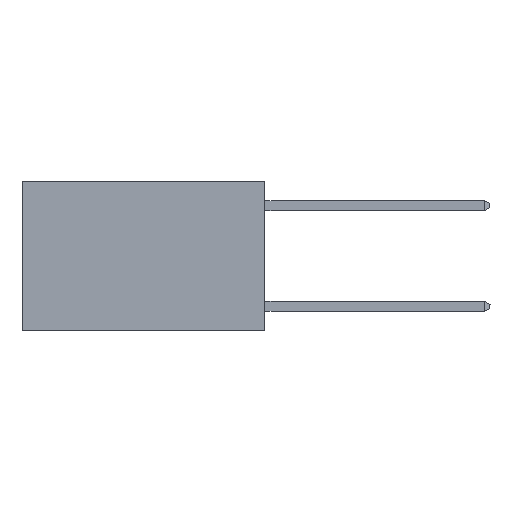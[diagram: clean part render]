
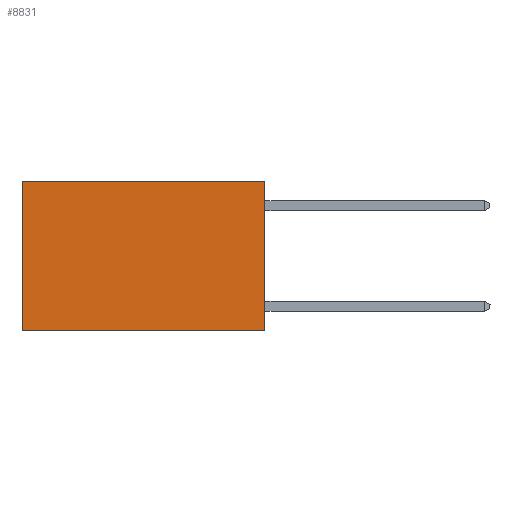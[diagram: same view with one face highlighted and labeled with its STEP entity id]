
A CAD part, left-side view. The second image highlights one B-rep face of the part: STEP entity #8831.
In plain terms, the highlighted planar face has unit normal (-1, 0, 0).
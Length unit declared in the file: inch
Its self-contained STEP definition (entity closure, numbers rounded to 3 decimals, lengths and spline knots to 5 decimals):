
#636 = DIRECTION ( 'NONE',  ( 1., 0., 0. ) ) ;
#891 = CARTESIAN_POINT ( 'NONE',  ( 0.2625, 0., 0. ) ) ;
#915 = VECTOR ( 'NONE', #25244, 39.37008 ) ;
#1284 = CARTESIAN_POINT ( 'NONE',  ( 0.2625, 0., 0. ) ) ;
#1459 = LINE ( 'NONE', #24831, #7036 ) ;
#3265 = CARTESIAN_POINT ( 'NONE',  ( 0.2625, 0.6, -0.37 ) ) ;
#4908 = EDGE_CURVE ( 'NONE', #12922, #5318, #19871, .T. ) ;
#5318 = VERTEX_POINT ( 'NONE', #16598 ) ;
#7036 = VECTOR ( 'NONE', #14418, 39.37008 ) ;
#7690 = ORIENTED_EDGE ( 'NONE', *, *, #24756, .T. ) ;
#8831 = ADVANCED_FACE ( 'NONE', ( #18918 ), #25833, .F. ) ;
#9711 = ORIENTED_EDGE ( 'NONE', *, *, #18122, .T. ) ;
#9890 = VECTOR ( 'NONE', #18022, 39.37008 ) ;
#11215 = EDGE_CURVE ( 'NONE', #5318, #19268, #1459, .T. ) ;
#12590 = DIRECTION ( 'NONE',  ( 0., 0., -1. ) ) ;
#12922 = VERTEX_POINT ( 'NONE', #1284 ) ;
#13351 = CARTESIAN_POINT ( 'NONE',  ( 0.2625, 0., 0. ) ) ;
#14124 = ORIENTED_EDGE ( 'NONE', *, *, #11215, .F. ) ;
#14418 = DIRECTION ( 'NONE',  ( 0., 1., 0. ) ) ;
#14811 = VECTOR ( 'NONE', #12590, 39.37008 ) ;
#15511 = DIRECTION ( 'NONE',  ( 0., 0., -1. ) ) ;
#15881 = CARTESIAN_POINT ( 'NONE',  ( 0.2625, 0., 0. ) ) ;
#16598 = CARTESIAN_POINT ( 'NONE',  ( 0.2625, 0., -0.37 ) ) ;
#18022 = DIRECTION ( 'NONE',  ( 0., 1., 0. ) ) ;
#18093 = AXIS2_PLACEMENT_3D ( 'NONE', #13351, #636, #15511 ) ;
#18122 = EDGE_CURVE ( 'NONE', #12922, #25478, #26632, .T. ) ;
#18724 = EDGE_LOOP ( 'NONE', ( #7690, #14124, #19756, #9711 ) ) ;
#18918 = FACE_OUTER_BOUND ( 'NONE', #18724, .T. ) ;
#19268 = VERTEX_POINT ( 'NONE', #3265 ) ;
#19756 = ORIENTED_EDGE ( 'NONE', *, *, #4908, .F. ) ;
#19871 = LINE ( 'NONE', #891, #915 ) ;
#20612 = CARTESIAN_POINT ( 'NONE',  ( 0.2625, 0.6, 0. ) ) ;
#21028 = CARTESIAN_POINT ( 'NONE',  ( 0.2625, 0.6, 0. ) ) ;
#21745 = LINE ( 'NONE', #21028, #14811 ) ;
#24756 = EDGE_CURVE ( 'NONE', #25478, #19268, #21745, .T. ) ;
#24831 = CARTESIAN_POINT ( 'NONE',  ( 0.2625, 0., -0.37 ) ) ;
#25244 = DIRECTION ( 'NONE',  ( 0., 0., -1. ) ) ;
#25478 = VERTEX_POINT ( 'NONE', #20612 ) ;
#25833 = PLANE ( 'NONE',  #18093 ) ;
#26632 = LINE ( 'NONE', #15881, #9890 ) ;
